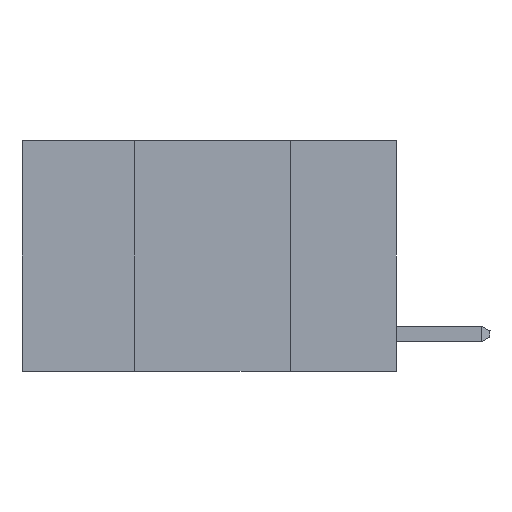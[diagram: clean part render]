
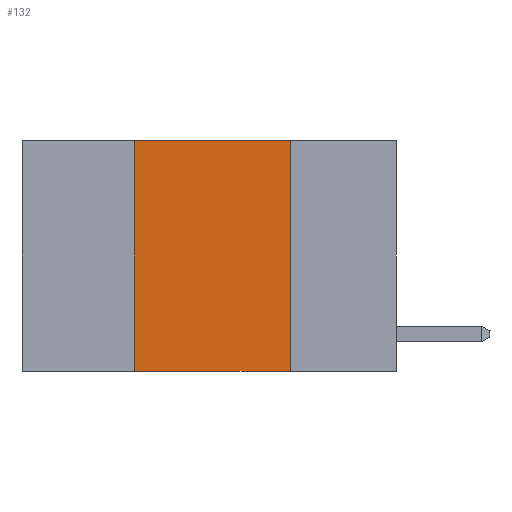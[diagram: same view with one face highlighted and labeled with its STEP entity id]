
A CAD part, left-side view. The second image highlights one B-rep face of the part: STEP entity #132.
In plain terms, the highlighted planar face has unit normal (-1, 0, 0).
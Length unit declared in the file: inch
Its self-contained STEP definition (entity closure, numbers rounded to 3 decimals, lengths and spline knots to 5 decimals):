
#132 = ADVANCED_FACE ( 'NONE', ( #903 ), #2428, .F. ) ;
#627 = DIRECTION ( 'NONE',  ( 1., 0., 0. ) ) ;
#903 = FACE_OUTER_BOUND ( 'NONE', #14272, .T. ) ;
#1551 = DIRECTION ( 'NONE',  ( 0., 0., -1. ) ) ;
#1806 = EDGE_CURVE ( 'NONE', #9497, #16821, #4826, .T. ) ;
#1972 = CARTESIAN_POINT ( 'NONE',  ( 0., 0.42, 0. ) ) ;
#2073 = DIRECTION ( 'NONE',  ( 0., 0., 1. ) ) ;
#2428 = PLANE ( 'NONE',  #10425 ) ;
#2904 = LINE ( 'NONE', #14202, #7963 ) ;
#3825 = DIRECTION ( 'NONE',  ( 0., 0., -1. ) ) ;
#3870 = CARTESIAN_POINT ( 'NONE',  ( 0., 0.17, -0.37 ) ) ;
#3899 = DIRECTION ( 'NONE',  ( 0., -1., 0. ) ) ;
#4212 = DIRECTION ( 'NONE',  ( 0., -1., 0. ) ) ;
#4826 = LINE ( 'NONE', #10171, #7243 ) ;
#5253 = ORIENTED_EDGE ( 'NONE', *, *, #1806, .F. ) ;
#5371 = VERTEX_POINT ( 'NONE', #11475 ) ;
#5563 = CARTESIAN_POINT ( 'NONE',  ( 0., 0.6, -0.37 ) ) ;
#7243 = VECTOR ( 'NONE', #1551, 39.37008 ) ;
#7623 = CARTESIAN_POINT ( 'NONE',  ( 0., 0.17, 0. ) ) ;
#7963 = VECTOR ( 'NONE', #4212, 39.37008 ) ;
#8613 = ORIENTED_EDGE ( 'NONE', *, *, #10149, .F. ) ;
#9180 = LINE ( 'NONE', #1972, #17436 ) ;
#9497 = VERTEX_POINT ( 'NONE', #7623 ) ;
#9504 = ORIENTED_EDGE ( 'NONE', *, *, #15767, .F. ) ;
#10149 = EDGE_CURVE ( 'NONE', #5371, #9497, #2904, .T. ) ;
#10171 = CARTESIAN_POINT ( 'NONE',  ( 0., 0.17, 0. ) ) ;
#10425 = AXIS2_PLACEMENT_3D ( 'NONE', #16596, #627, #3825 ) ;
#11213 = EDGE_CURVE ( 'NONE', #11616, #16821, #16684, .T. ) ;
#11475 = CARTESIAN_POINT ( 'NONE',  ( 0., 0.42, 0. ) ) ;
#11616 = VERTEX_POINT ( 'NONE', #15509 ) ;
#14202 = CARTESIAN_POINT ( 'NONE',  ( 0., 0.6, 0. ) ) ;
#14272 = EDGE_LOOP ( 'NONE', ( #5253, #8613, #9504, #15388 ) ) ;
#15388 = ORIENTED_EDGE ( 'NONE', *, *, #11213, .T. ) ;
#15439 = VECTOR ( 'NONE', #3899, 39.37008 ) ;
#15509 = CARTESIAN_POINT ( 'NONE',  ( 0., 0.42, -0.37 ) ) ;
#15767 = EDGE_CURVE ( 'NONE', #11616, #5371, #9180, .T. ) ;
#16596 = CARTESIAN_POINT ( 'NONE',  ( 0., 0.6, 0. ) ) ;
#16684 = LINE ( 'NONE', #5563, #15439 ) ;
#16821 = VERTEX_POINT ( 'NONE', #3870 ) ;
#17436 = VECTOR ( 'NONE', #2073, 39.37008 ) ;
